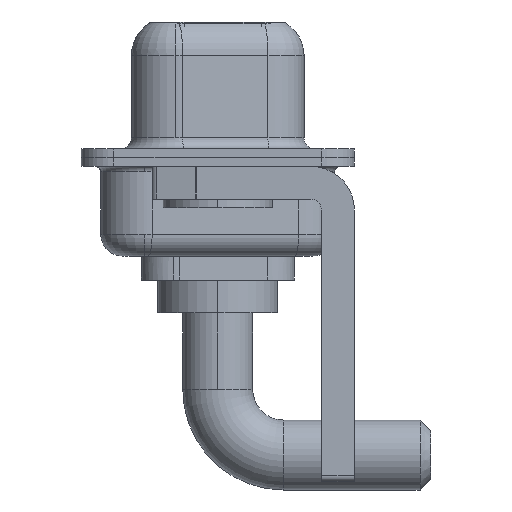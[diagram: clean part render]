
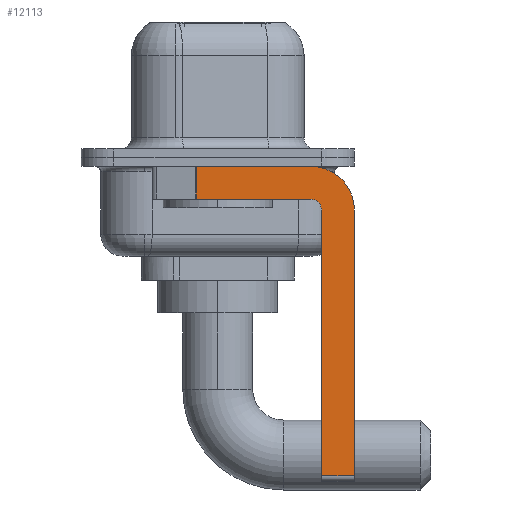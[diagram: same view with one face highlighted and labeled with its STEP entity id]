
A CAD part, left-side view. The second image highlights one B-rep face of the part: STEP entity #12113.
In plain terms, the highlighted planar face has unit normal (-1, 0, 0).
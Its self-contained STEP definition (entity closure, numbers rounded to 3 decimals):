
#79 = VECTOR ( 'NONE', #7225, 1000. ) ;
#1017 = DIRECTION ( 'NONE',  ( 1., 0., 0. ) ) ;
#1041 = LINE ( 'NONE', #7376, #3158 ) ;
#1081 = CARTESIAN_POINT ( 'NONE',  ( -2.9, 0.978, -1.9 ) ) ;
#1085 = LINE ( 'NONE', #9218, #4702 ) ;
#1161 = LINE ( 'NONE', #13083, #11718 ) ;
#1208 = DIRECTION ( 'NONE',  ( 1., 0., 0. ) ) ;
#1622 = ORIENTED_EDGE ( 'NONE', *, *, #12782, .F. ) ;
#2413 = CARTESIAN_POINT ( 'NONE',  ( -2.9, -4.25, -0.4 ) ) ;
#2652 = EDGE_CURVE ( 'NONE', #10076, #12085, #1161, .T. ) ;
#2664 = VERTEX_POINT ( 'NONE', #10020 ) ;
#3140 = VECTOR ( 'NONE', #7571, 1000. ) ;
#3158 = VECTOR ( 'NONE', #7445, 1000. ) ;
#3650 = VERTEX_POINT ( 'NONE', #4278 ) ;
#3851 = CARTESIAN_POINT ( 'NONE',  ( -2.9, 0.978, -1.9 ) ) ;
#4017 = CARTESIAN_POINT ( 'NONE',  ( -2.9, -4.25, -1.9 ) ) ;
#4278 = CARTESIAN_POINT ( 'NONE',  ( -2.9, -6.25, -14.55 ) ) ;
#4412 = EDGE_CURVE ( 'NONE', #7928, #9311, #5519, .T. ) ;
#4521 = DIRECTION ( 'NONE',  ( 0., -1., 0. ) ) ;
#4600 = VERTEX_POINT ( 'NONE', #7801 ) ;
#4702 = VECTOR ( 'NONE', #13429, 1000. ) ;
#4786 = EDGE_LOOP ( 'NONE', ( #13281, #7707, #7908, #8397, #1622, #9725, #8622, #9921 ) ) ;
#4977 = CARTESIAN_POINT ( 'NONE',  ( -2.9, -4.25, -14.55 ) ) ;
#5230 = FACE_OUTER_BOUND ( 'NONE', #4786, .T. ) ;
#5397 = DIRECTION ( 'NONE',  ( 0., 0., 1. ) ) ;
#5519 = LINE ( 'NONE', #9652, #5684 ) ;
#5684 = VECTOR ( 'NONE', #4521, 1000. ) ;
#5995 = LINE ( 'NONE', #4977, #79 ) ;
#6850 = AXIS2_PLACEMENT_3D ( 'NONE', #11478, #8628, #5397 ) ;
#7021 = AXIS2_PLACEMENT_3D ( 'NONE', #7549, #1208, #11778 ) ;
#7225 = DIRECTION ( 'NONE',  ( 0., -1., 0. ) ) ;
#7376 = CARTESIAN_POINT ( 'NONE',  ( -2.9, -4.75, -14.8 ) ) ;
#7445 = DIRECTION ( 'NONE',  ( 0., 0., 1. ) ) ;
#7519 = AXIS2_PLACEMENT_3D ( 'NONE', #10368, #1017, #9415 ) ;
#7549 = CARTESIAN_POINT ( 'NONE',  ( -2.9, -4.25, -2.4 ) ) ;
#7571 = DIRECTION ( 'NONE',  ( 0., 0., -1. ) ) ;
#7707 = ORIENTED_EDGE ( 'NONE', *, *, #10488, .T. ) ;
#7801 = CARTESIAN_POINT ( 'NONE',  ( -2.9, -6.25, -2.4 ) ) ;
#7908 = ORIENTED_EDGE ( 'NONE', *, *, #2652, .F. ) ;
#7928 = VERTEX_POINT ( 'NONE', #11415 ) ;
#8379 = CIRCLE ( 'NONE', #6850, 0.5 ) ;
#8397 = ORIENTED_EDGE ( 'NONE', *, *, #9826, .F. ) ;
#8622 = ORIENTED_EDGE ( 'NONE', *, *, #13353, .F. ) ;
#8628 = DIRECTION ( 'NONE',  ( -1., 0., 0. ) ) ;
#8682 = LINE ( 'NONE', #3851, #3140 ) ;
#8757 = EDGE_CURVE ( 'NONE', #9311, #4600, #12915, .T. ) ;
#9218 = CARTESIAN_POINT ( 'NONE',  ( -2.9, -6.25, -2.4 ) ) ;
#9311 = VERTEX_POINT ( 'NONE', #2413 ) ;
#9415 = DIRECTION ( 'NONE',  ( 0., 0., -1. ) ) ;
#9652 = CARTESIAN_POINT ( 'NONE',  ( -2.9, 3., -0.4 ) ) ;
#9725 = ORIENTED_EDGE ( 'NONE', *, *, #11411, .T. ) ;
#9826 = EDGE_CURVE ( 'NONE', #13337, #10076, #8379, .T. ) ;
#9921 = ORIENTED_EDGE ( 'NONE', *, *, #8757, .F. ) ;
#10020 = CARTESIAN_POINT ( 'NONE',  ( -2.9, -4.75, -14.55 ) ) ;
#10076 = VERTEX_POINT ( 'NONE', #4017 ) ;
#10368 = CARTESIAN_POINT ( 'NONE',  ( -2.9, -4.25, -2.4 ) ) ;
#10488 = EDGE_CURVE ( 'NONE', #7928, #12085, #8682, .T. ) ;
#11411 = EDGE_CURVE ( 'NONE', #2664, #3650, #5995, .T. ) ;
#11415 = CARTESIAN_POINT ( 'NONE',  ( -2.9, 0.978, -0.4 ) ) ;
#11478 = CARTESIAN_POINT ( 'NONE',  ( -2.9, -4.25, -2.4 ) ) ;
#11718 = VECTOR ( 'NONE', #12946, 1000. ) ;
#11778 = DIRECTION ( 'NONE',  ( 0., 0., -1. ) ) ;
#12085 = VERTEX_POINT ( 'NONE', #1081 ) ;
#12113 = ADVANCED_FACE ( 'NONE', ( #5230 ), #12336, .F. ) ;
#12336 = PLANE ( 'NONE',  #7519 ) ;
#12782 = EDGE_CURVE ( 'NONE', #2664, #13337, #1041, .T. ) ;
#12915 = CIRCLE ( 'NONE', #7021, 2. ) ;
#12946 = DIRECTION ( 'NONE',  ( 0., 1., 0. ) ) ;
#13083 = CARTESIAN_POINT ( 'NONE',  ( -2.9, -4.25, -1.9 ) ) ;
#13281 = ORIENTED_EDGE ( 'NONE', *, *, #4412, .F. ) ;
#13337 = VERTEX_POINT ( 'NONE', #13358 ) ;
#13353 = EDGE_CURVE ( 'NONE', #4600, #3650, #1085, .T. ) ;
#13358 = CARTESIAN_POINT ( 'NONE',  ( -2.9, -4.75, -2.4 ) ) ;
#13429 = DIRECTION ( 'NONE',  ( 0., 0., -1. ) ) ;
